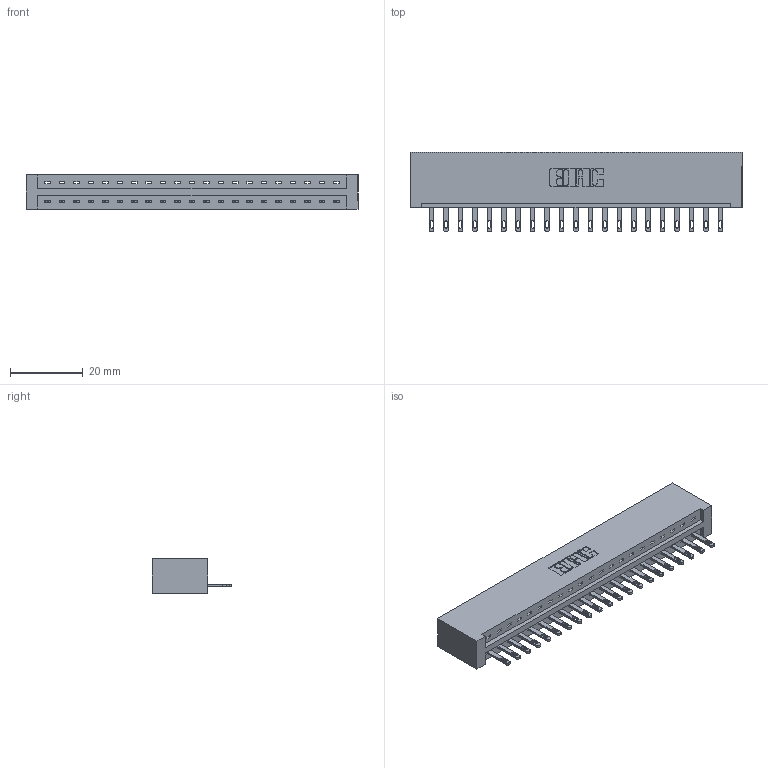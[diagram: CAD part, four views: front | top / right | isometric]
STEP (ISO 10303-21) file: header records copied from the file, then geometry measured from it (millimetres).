
FILE_DESCRIPTION (( 'STEP AP203' ), '1' );
FILE_NAME ('887-021-500-101.STEP', '2020-09-20T18:19:42', ( '' ), ( '' ), 'SwSTEP 2.0', 'SolidWorks 2020', '' );
FILE_SCHEMA (( 'CONFIG_CONTROL_DESIGN' ));
Length unit declared in the file: inch
Products named in the file (3): 887-021-500-101; 345-292-001_345-293-100; 837 Part_No Mounting Lugs
Assembly tree (22 placements, depth 2):
  887-021-500-101
    837 Part_No Mounting Lugs
    345-292-001_345-293-100  x21
Bounding box: 91.08 x 21.85 x 9.4 mm (x, y, z)
Volume: 9955.6 mm3; surface area: 10201.6 mm2
Topology: 22 solids, 22 shells, 1324 faces, 4067 edges, 2710 vertices
Faces by surface type: plane 906, cylinder 418
Entity records: 17979 total; most frequent: CARTESIAN_POINT 3137, ORIENTED_EDGE 3094, DIRECTION 2677, EDGE_CURVE 1547, VECTOR 1423, LINE 1423, VERTEX_POINT 1030, AXIS2_PLACEMENT_3D 627
